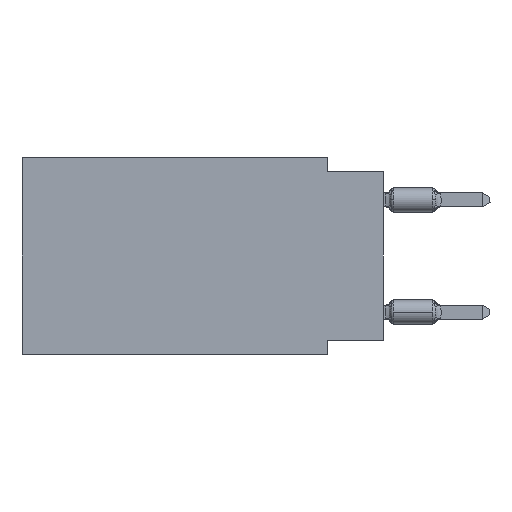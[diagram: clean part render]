
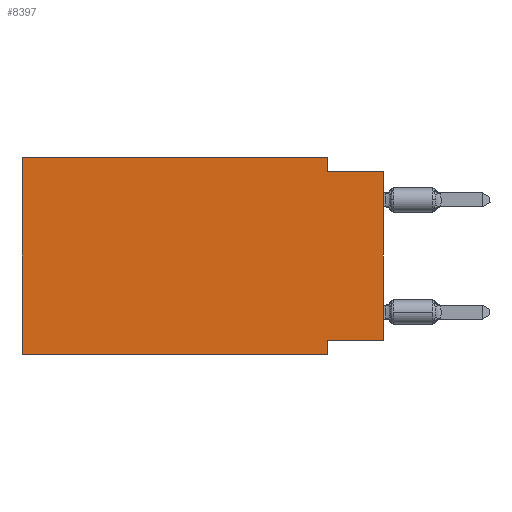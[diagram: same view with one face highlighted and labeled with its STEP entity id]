
A CAD part, left-side view. The second image highlights one B-rep face of the part: STEP entity #8397.
In plain terms, the highlighted planar face has unit normal (-1, 0, 0).
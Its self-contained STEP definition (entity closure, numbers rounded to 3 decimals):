
#93 = LINE ( 'NONE', #7168, #17868 ) ;
#756 = ORIENTED_EDGE ( 'NONE', *, *, #17705, .F. ) ;
#1370 = FACE_OUTER_BOUND ( 'NONE', #7858, .T. ) ;
#2486 = DIRECTION ( 'NONE',  ( 0., 0., -1. ) ) ;
#3483 = VECTOR ( 'NONE', #11724, 1000. ) ;
#3695 = CARTESIAN_POINT ( 'NONE',  ( 0., 16.383, 0. ) ) ;
#5584 = CARTESIAN_POINT ( 'NONE',  ( 0., 2.54, -8.255 ) ) ;
#5869 = ORIENTED_EDGE ( 'NONE', *, *, #26680, .F. ) ;
#6222 = ORIENTED_EDGE ( 'NONE', *, *, #21689, .F. ) ;
#6301 = EDGE_CURVE ( 'NONE', #8387, #25733, #21268, .T. ) ;
#6353 = VECTOR ( 'NONE', #25476, 1000. ) ;
#6742 = LINE ( 'NONE', #18174, #16305 ) ;
#6759 = ORIENTED_EDGE ( 'NONE', *, *, #27911, .F. ) ;
#7168 = CARTESIAN_POINT ( 'NONE',  ( 0., 2.54, -8.89 ) ) ;
#7175 = ORIENTED_EDGE ( 'NONE', *, *, #27056, .F. ) ;
#7858 = EDGE_LOOP ( 'NONE', ( #9595, #6759, #27386, #7175, #6222, #21128, #5869, #756 ) ) ;
#7886 = CARTESIAN_POINT ( 'NONE',  ( 0., 16.383, -8.89 ) ) ;
#7918 = LINE ( 'NONE', #21602, #20972 ) ;
#8086 = VERTEX_POINT ( 'NONE', #15236 ) ;
#8342 = VECTOR ( 'NONE', #9997, 1000. ) ;
#8387 = VERTEX_POINT ( 'NONE', #10688 ) ;
#8397 = ADVANCED_FACE ( 'NONE', ( #1370 ), #14900, .F. ) ;
#9520 = VECTOR ( 'NONE', #20909, 1000. ) ;
#9595 = ORIENTED_EDGE ( 'NONE', *, *, #20382, .T. ) ;
#9843 = CARTESIAN_POINT ( 'NONE',  ( 0., 2.54, 0. ) ) ;
#9997 = DIRECTION ( 'NONE',  ( 0., 0., -1. ) ) ;
#10096 = CARTESIAN_POINT ( 'NONE',  ( 0., 16.383, -8.89 ) ) ;
#10688 = CARTESIAN_POINT ( 'NONE',  ( 0., 2.54, 0. ) ) ;
#11313 = LINE ( 'NONE', #27541, #9520 ) ;
#11724 = DIRECTION ( 'NONE',  ( 0., -1., 0. ) ) ;
#12038 = VERTEX_POINT ( 'NONE', #3695 ) ;
#14119 = CARTESIAN_POINT ( 'NONE',  ( 0., 0., -0.635 ) ) ;
#14678 = DIRECTION ( 'NONE',  ( 0., 1., 0. ) ) ;
#14900 = PLANE ( 'NONE',  #18048 ) ;
#15236 = CARTESIAN_POINT ( 'NONE',  ( 0., 2.54, -8.89 ) ) ;
#15447 = EDGE_CURVE ( 'NONE', #25635, #8086, #28490, .T. ) ;
#15518 = CARTESIAN_POINT ( 'NONE',  ( 0., 2.54, -0.635 ) ) ;
#15880 = VERTEX_POINT ( 'NONE', #5584 ) ;
#16241 = LINE ( 'NONE', #14119, #3483 ) ;
#16305 = VECTOR ( 'NONE', #29317, 1000. ) ;
#17056 = DIRECTION ( 'NONE',  ( 0., -1., 0. ) ) ;
#17620 = DIRECTION ( 'NONE',  ( 1., 0., 0. ) ) ;
#17705 = EDGE_CURVE ( 'NONE', #19294, #15880, #7918, .T. ) ;
#17868 = VECTOR ( 'NONE', #2486, 1000. ) ;
#18048 = AXIS2_PLACEMENT_3D ( 'NONE', #24682, #17620, #28893 ) ;
#18174 = CARTESIAN_POINT ( 'NONE',  ( 0., 16.383, 0. ) ) ;
#18273 = CARTESIAN_POINT ( 'NONE',  ( 0., 16.383, 0. ) ) ;
#19294 = VERTEX_POINT ( 'NONE', #26743 ) ;
#20382 = EDGE_CURVE ( 'NONE', #19294, #21044, #11313, .T. ) ;
#20909 = DIRECTION ( 'NONE',  ( 0., 0., 1. ) ) ;
#20972 = VECTOR ( 'NONE', #14678, 1000. ) ;
#21044 = VERTEX_POINT ( 'NONE', #28836 ) ;
#21128 = ORIENTED_EDGE ( 'NONE', *, *, #15447, .T. ) ;
#21268 = LINE ( 'NONE', #9843, #8342 ) ;
#21602 = CARTESIAN_POINT ( 'NONE',  ( 0., 0., -8.255 ) ) ;
#21689 = EDGE_CURVE ( 'NONE', #25635, #12038, #6742, .T. ) ;
#22953 = LINE ( 'NONE', #18273, #6353 ) ;
#24682 = CARTESIAN_POINT ( 'NONE',  ( 0., 16.383, 0. ) ) ;
#25476 = DIRECTION ( 'NONE',  ( 0., -1., 0. ) ) ;
#25635 = VERTEX_POINT ( 'NONE', #10096 ) ;
#25733 = VERTEX_POINT ( 'NONE', #15518 ) ;
#26247 = VECTOR ( 'NONE', #17056, 1000. ) ;
#26680 = EDGE_CURVE ( 'NONE', #15880, #8086, #93, .T. ) ;
#26743 = CARTESIAN_POINT ( 'NONE',  ( 0., 0., -8.255 ) ) ;
#27056 = EDGE_CURVE ( 'NONE', #12038, #8387, #22953, .T. ) ;
#27386 = ORIENTED_EDGE ( 'NONE', *, *, #6301, .F. ) ;
#27541 = CARTESIAN_POINT ( 'NONE',  ( 0., 0., 0. ) ) ;
#27911 = EDGE_CURVE ( 'NONE', #25733, #21044, #16241, .T. ) ;
#28490 = LINE ( 'NONE', #7886, #26247 ) ;
#28836 = CARTESIAN_POINT ( 'NONE',  ( 0., 0., -0.635 ) ) ;
#28893 = DIRECTION ( 'NONE',  ( 0., 0., -1. ) ) ;
#29317 = DIRECTION ( 'NONE',  ( 0., 0., 1. ) ) ;
